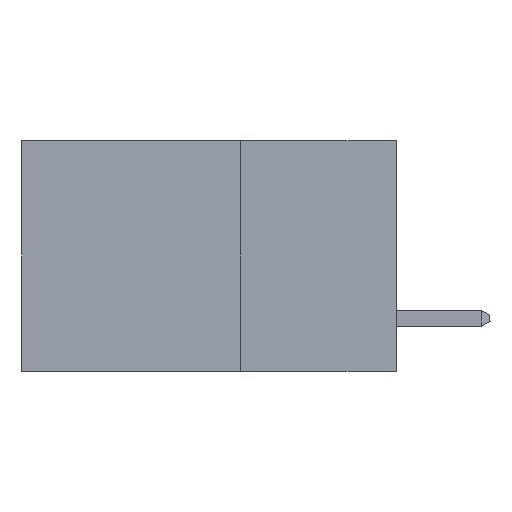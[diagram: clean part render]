
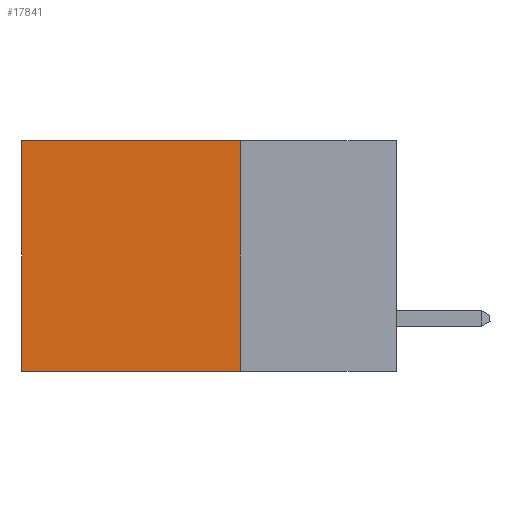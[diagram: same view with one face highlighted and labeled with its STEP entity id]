
A CAD part, left-side view. The second image highlights one B-rep face of the part: STEP entity #17841.
In plain terms, the highlighted planar face has unit normal (-1, 0, 0).
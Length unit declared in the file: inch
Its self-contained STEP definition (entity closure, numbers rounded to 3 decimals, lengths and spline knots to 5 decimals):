
#113 = CARTESIAN_POINT ( 'NONE',  ( 0.298, 0.25, 0. ) ) ;
#1389 = FACE_OUTER_BOUND ( 'NONE', #4170, .T. ) ;
#2206 = LINE ( 'NONE', #5611, #13905 ) ;
#4170 = EDGE_LOOP ( 'NONE', ( #14216, #24921, #20468, #4665 ) ) ;
#4665 = ORIENTED_EDGE ( 'NONE', *, *, #21518, .T. ) ;
#5611 = CARTESIAN_POINT ( 'NONE',  ( 0.298, 0.25, 0. ) ) ;
#6537 = VECTOR ( 'NONE', #26706, 39.37008 ) ;
#7177 = EDGE_CURVE ( 'NONE', #14676, #23881, #16922, .T. ) ;
#7574 = VERTEX_POINT ( 'NONE', #27900 ) ;
#9165 = AXIS2_PLACEMENT_3D ( 'NONE', #12323, #28410, #14643 ) ;
#9301 = VECTOR ( 'NONE', #14108, 39.37008 ) ;
#12323 = CARTESIAN_POINT ( 'NONE',  ( 0.298, 0.25, 0. ) ) ;
#12764 = DIRECTION ( 'NONE',  ( 0., 1., 0. ) ) ;
#12968 = CARTESIAN_POINT ( 'NONE',  ( 0.298, 0.6, 0. ) ) ;
#13905 = VECTOR ( 'NONE', #24074, 39.37008 ) ;
#14050 = VERTEX_POINT ( 'NONE', #14786 ) ;
#14108 = DIRECTION ( 'NONE',  ( 0., 1., 0. ) ) ;
#14216 = ORIENTED_EDGE ( 'NONE', *, *, #28572, .T. ) ;
#14643 = DIRECTION ( 'NONE',  ( 0., 0., -1. ) ) ;
#14676 = VERTEX_POINT ( 'NONE', #26170 ) ;
#14786 = CARTESIAN_POINT ( 'NONE',  ( 0.298, 0.25, 0. ) ) ;
#14876 = CARTESIAN_POINT ( 'NONE',  ( 0.298, 0.6, -0.37 ) ) ;
#16223 = LINE ( 'NONE', #113, #9301 ) ;
#16922 = LINE ( 'NONE', #28832, #22342 ) ;
#17841 = ADVANCED_FACE ( 'NONE', ( #1389 ), #21473, .F. ) ;
#19543 = LINE ( 'NONE', #12968, #6537 ) ;
#20468 = ORIENTED_EDGE ( 'NONE', *, *, #26682, .F. ) ;
#21473 = PLANE ( 'NONE',  #9165 ) ;
#21518 = EDGE_CURVE ( 'NONE', #14050, #7574, #16223, .T. ) ;
#22342 = VECTOR ( 'NONE', #12764, 39.37008 ) ;
#23881 = VERTEX_POINT ( 'NONE', #14876 ) ;
#24074 = DIRECTION ( 'NONE',  ( 0., 0., -1. ) ) ;
#24921 = ORIENTED_EDGE ( 'NONE', *, *, #7177, .F. ) ;
#26170 = CARTESIAN_POINT ( 'NONE',  ( 0.298, 0.25, -0.37 ) ) ;
#26682 = EDGE_CURVE ( 'NONE', #14050, #14676, #2206, .T. ) ;
#26706 = DIRECTION ( 'NONE',  ( 0., 0., -1. ) ) ;
#27900 = CARTESIAN_POINT ( 'NONE',  ( 0.298, 0.6, 0. ) ) ;
#28410 = DIRECTION ( 'NONE',  ( 1., 0., 0. ) ) ;
#28572 = EDGE_CURVE ( 'NONE', #7574, #23881, #19543, .T. ) ;
#28832 = CARTESIAN_POINT ( 'NONE',  ( 0.298, 0.25, -0.37 ) ) ;
